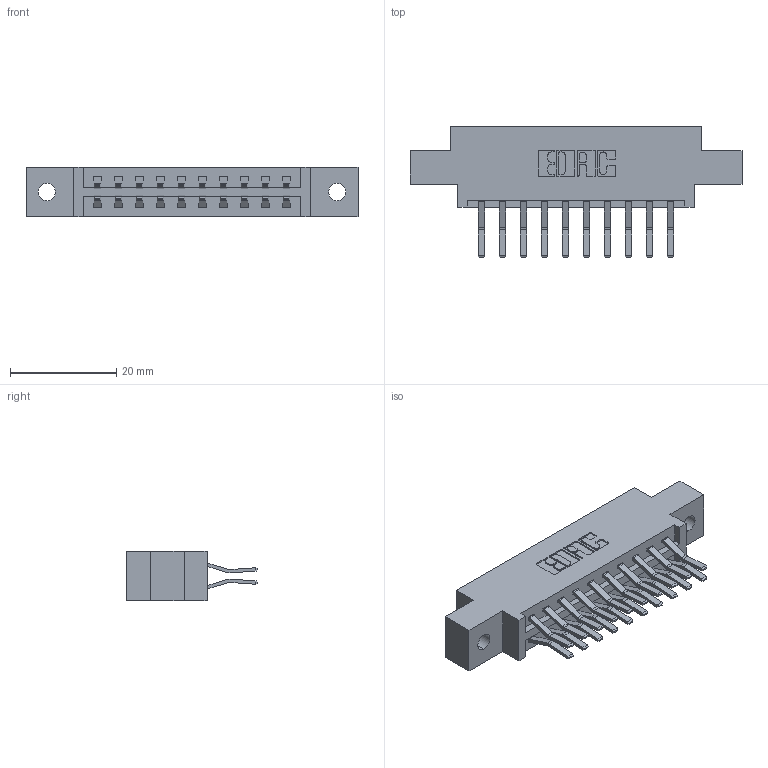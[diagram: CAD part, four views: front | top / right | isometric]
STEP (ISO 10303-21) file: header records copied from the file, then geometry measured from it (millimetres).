
FILE_DESCRIPTION (( 'STEP AP203' ), '1' );
FILE_NAME ('387-020-560-802.STEP', '2019-10-16T16:10:53', ( '' ), ( '' ), 'SwSTEP 2.0', 'SolidWorks 2016', '' );
FILE_SCHEMA (( 'CONFIG_CONTROL_DESIGN' ));
Length unit declared in the file: inch
Products named in the file (3): 337 Part_0.170 Offset - 0.128 Dia; 345-292-001_560 Tail; 387-020-560-802
Assembly tree (21 placements, depth 2):
  387-020-560-802
    337 Part_0.170 Offset - 0.128 Dia
    345-292-001_560 Tail  x20
Bounding box: 62.64 x 24.78 x 9.4 mm (x, y, z)
Volume: 6152.1 mm3; surface area: 6858.6 mm2
Topology: 21 solids, 21 shells, 1238 faces, 3663 edges, 2414 vertices
Faces by surface type: plane 834, cylinder 404
Entity records: 12115 total; most frequent: CARTESIAN_POINT 2070, ORIENTED_EDGE 2006, DIRECTION 1823, EDGE_CURVE 1003, VECTOR 871, LINE 871, VERTEX_POINT 666, AXIS2_PLACEMENT_3D 476
